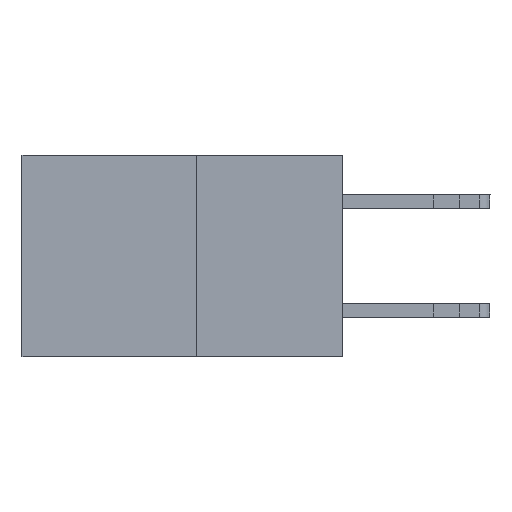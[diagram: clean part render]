
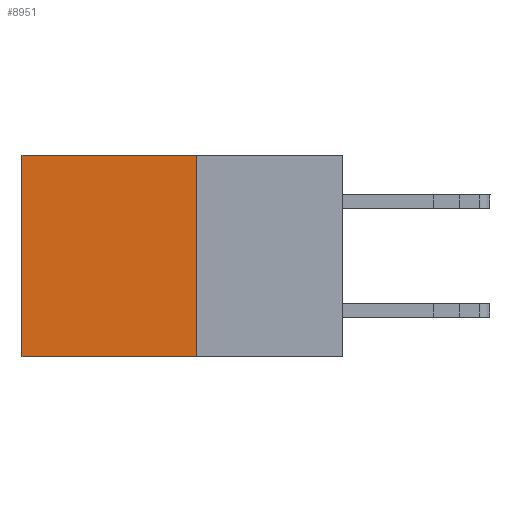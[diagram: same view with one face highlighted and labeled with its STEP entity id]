
A CAD part, left-side view. The second image highlights one B-rep face of the part: STEP entity #8951.
In plain terms, the highlighted planar face has unit normal (-1, 0, 0).
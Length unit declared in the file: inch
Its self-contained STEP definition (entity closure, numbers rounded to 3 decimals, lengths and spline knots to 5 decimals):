
#851 = EDGE_CURVE ( 'NONE', #7712, #3029, #9891, .T. ) ;
#1270 = LINE ( 'NONE', #11338, #5466 ) ;
#1881 = CARTESIAN_POINT ( 'NONE',  ( 0.277, 0.27, -0.37 ) ) ;
#2331 = FACE_OUTER_BOUND ( 'NONE', #10460, .T. ) ;
#3029 = VERTEX_POINT ( 'NONE', #4496 ) ;
#3172 = VERTEX_POINT ( 'NONE', #3679 ) ;
#3439 = PLANE ( 'NONE',  #9038 ) ;
#3622 = LINE ( 'NONE', #7279, #9820 ) ;
#3654 = DIRECTION ( 'NONE',  ( 0., 0., -1. ) ) ;
#3679 = CARTESIAN_POINT ( 'NONE',  ( 0.277, 0.27, 0. ) ) ;
#4319 = ORIENTED_EDGE ( 'NONE', *, *, #851, .F. ) ;
#4443 = DIRECTION ( 'NONE',  ( 0., 1., 0. ) ) ;
#4496 = CARTESIAN_POINT ( 'NONE',  ( 0.277, 0.59, -0.37 ) ) ;
#4974 = VERTEX_POINT ( 'NONE', #11425 ) ;
#5008 = DIRECTION ( 'NONE',  ( 0., 0., -1. ) ) ;
#5402 = EDGE_CURVE ( 'NONE', #4974, #3029, #1270, .T. ) ;
#5466 = VECTOR ( 'NONE', #13807, 39.37008 ) ;
#5581 = DIRECTION ( 'NONE',  ( 1., 0., 0. ) ) ;
#6948 = CARTESIAN_POINT ( 'NONE',  ( 0.277, 0.27, -0.37 ) ) ;
#7279 = CARTESIAN_POINT ( 'NONE',  ( 0.277, 0.27, -0.37 ) ) ;
#7712 = VERTEX_POINT ( 'NONE', #8456 ) ;
#8330 = VECTOR ( 'NONE', #9815, 39.37008 ) ;
#8456 = CARTESIAN_POINT ( 'NONE',  ( 0.277, 0.27, -0.37 ) ) ;
#8951 = ADVANCED_FACE ( 'NONE', ( #2331 ), #3439, .F. ) ;
#9038 = AXIS2_PLACEMENT_3D ( 'NONE', #6948, #5581, #3654 ) ;
#9815 = DIRECTION ( 'NONE',  ( 0., 1., 0. ) ) ;
#9820 = VECTOR ( 'NONE', #5008, 39.37008 ) ;
#9868 = CARTESIAN_POINT ( 'NONE',  ( 0.277, 0.27, 0. ) ) ;
#9891 = LINE ( 'NONE', #1881, #8330 ) ;
#9987 = ORIENTED_EDGE ( 'NONE', *, *, #12474, .T. ) ;
#10030 = EDGE_CURVE ( 'NONE', #3172, #7712, #3622, .T. ) ;
#10319 = VECTOR ( 'NONE', #4443, 39.37008 ) ;
#10460 = EDGE_LOOP ( 'NONE', ( #13953, #4319, #11619, #9987 ) ) ;
#11338 = CARTESIAN_POINT ( 'NONE',  ( 0.277, 0.59, -0.37 ) ) ;
#11425 = CARTESIAN_POINT ( 'NONE',  ( 0.277, 0.59, 0. ) ) ;
#11619 = ORIENTED_EDGE ( 'NONE', *, *, #10030, .F. ) ;
#12070 = LINE ( 'NONE', #9868, #10319 ) ;
#12474 = EDGE_CURVE ( 'NONE', #3172, #4974, #12070, .T. ) ;
#13807 = DIRECTION ( 'NONE',  ( 0., 0., -1. ) ) ;
#13953 = ORIENTED_EDGE ( 'NONE', *, *, #5402, .T. ) ;
